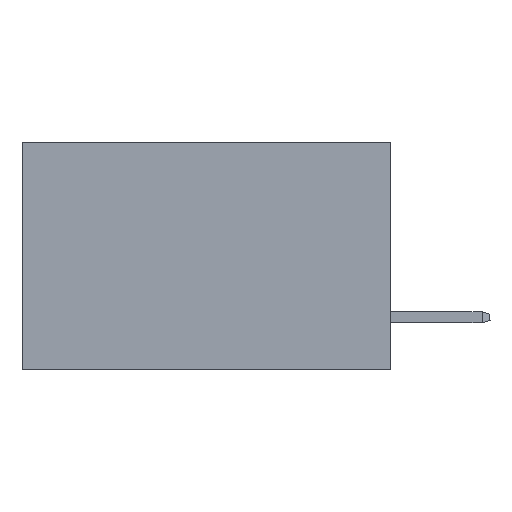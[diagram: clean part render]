
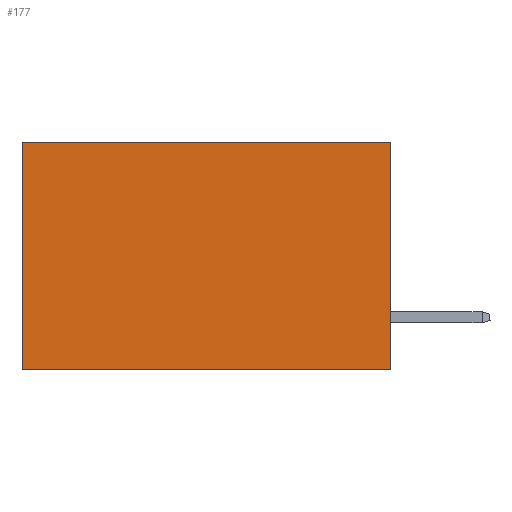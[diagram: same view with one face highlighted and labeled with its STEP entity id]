
A CAD part, left-side view. The second image highlights one B-rep face of the part: STEP entity #177.
In plain terms, the highlighted planar face has unit normal (-1, 0, 0).
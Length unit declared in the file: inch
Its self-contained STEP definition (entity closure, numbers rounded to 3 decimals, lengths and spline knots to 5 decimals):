
#177 = ADVANCED_FACE ( 'NONE', ( #3077 ), #1806, .F. ) ;
#1687 = EDGE_LOOP ( 'NONE', ( #17608, #26058, #20381, #23425 ) ) ;
#1806 = PLANE ( 'NONE',  #23411 ) ;
#3077 = FACE_OUTER_BOUND ( 'NONE', #1687, .T. ) ;
#3547 = CARTESIAN_POINT ( 'NONE',  ( 0.2875, 0., 0. ) ) ;
#4028 = DIRECTION ( 'NONE',  ( 1., 0., 0. ) ) ;
#4213 = DIRECTION ( 'NONE',  ( 0., 0., -1. ) ) ;
#4236 = LINE ( 'NONE', #13846, #22622 ) ;
#5067 = VERTEX_POINT ( 'NONE', #20804 ) ;
#5581 = EDGE_CURVE ( 'NONE', #9407, #10190, #4236, .T. ) ;
#5675 = LINE ( 'NONE', #21100, #19304 ) ;
#6086 = DIRECTION ( 'NONE',  ( 0., 0., -1. ) ) ;
#7804 = DIRECTION ( 'NONE',  ( 0., 0., -1. ) ) ;
#8094 = EDGE_CURVE ( 'NONE', #9407, #5067, #10079, .T. ) ;
#8317 = DIRECTION ( 'NONE',  ( 0., 1., 0. ) ) ;
#9407 = VERTEX_POINT ( 'NONE', #19747 ) ;
#10079 = LINE ( 'NONE', #3547, #26844 ) ;
#10190 = VERTEX_POINT ( 'NONE', #15953 ) ;
#10314 = CARTESIAN_POINT ( 'NONE',  ( 0.2875, 0.6, 0. ) ) ;
#13846 = CARTESIAN_POINT ( 'NONE',  ( 0.2875, 0., 0. ) ) ;
#14952 = CARTESIAN_POINT ( 'NONE',  ( 0.2875, 0., 0. ) ) ;
#15275 = VECTOR ( 'NONE', #7804, 39.37008 ) ;
#15492 = EDGE_CURVE ( 'NONE', #5067, #23977, #5675, .T. ) ;
#15953 = CARTESIAN_POINT ( 'NONE',  ( 0.2875, 0.6, 0. ) ) ;
#15993 = DIRECTION ( 'NONE',  ( 0., 1., 0. ) ) ;
#16374 = EDGE_CURVE ( 'NONE', #10190, #23977, #23300, .T. ) ;
#17608 = ORIENTED_EDGE ( 'NONE', *, *, #16374, .T. ) ;
#19304 = VECTOR ( 'NONE', #8317, 39.37008 ) ;
#19747 = CARTESIAN_POINT ( 'NONE',  ( 0.2875, 0., 0. ) ) ;
#19795 = CARTESIAN_POINT ( 'NONE',  ( 0.2875, 0.6, -0.37 ) ) ;
#20381 = ORIENTED_EDGE ( 'NONE', *, *, #8094, .F. ) ;
#20804 = CARTESIAN_POINT ( 'NONE',  ( 0.2875, 0., -0.37 ) ) ;
#21100 = CARTESIAN_POINT ( 'NONE',  ( 0.2875, 0., -0.37 ) ) ;
#22622 = VECTOR ( 'NONE', #15993, 39.37008 ) ;
#23300 = LINE ( 'NONE', #10314, #15275 ) ;
#23411 = AXIS2_PLACEMENT_3D ( 'NONE', #14952, #4028, #4213 ) ;
#23425 = ORIENTED_EDGE ( 'NONE', *, *, #5581, .T. ) ;
#23977 = VERTEX_POINT ( 'NONE', #19795 ) ;
#26058 = ORIENTED_EDGE ( 'NONE', *, *, #15492, .F. ) ;
#26844 = VECTOR ( 'NONE', #6086, 39.37008 ) ;
